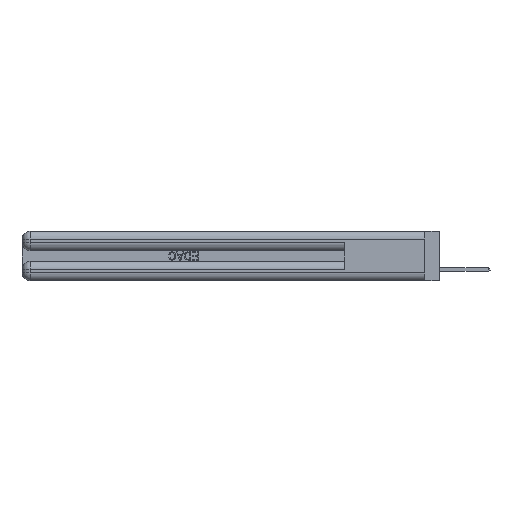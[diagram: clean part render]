
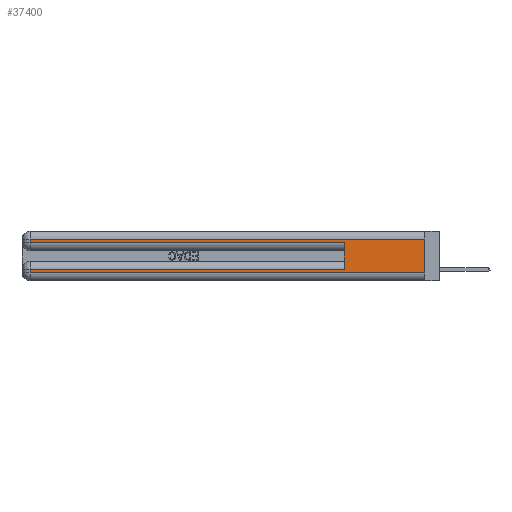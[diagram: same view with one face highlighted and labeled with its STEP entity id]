
A CAD part, left-side view. The second image highlights one B-rep face of the part: STEP entity #37400.
In plain terms, the highlighted planar face has unit normal (-1, 0, 0).
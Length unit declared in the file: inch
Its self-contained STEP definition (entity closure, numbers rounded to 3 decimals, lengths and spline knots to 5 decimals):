
#959 = FACE_OUTER_BOUND ( 'NONE', #41327, .T. ) ;
#1634 = CARTESIAN_POINT ( 'NONE',  ( 0., 2.94, 0.085 ) ) ;
#2557 = DIRECTION ( 'NONE',  ( 0., -1., 0. ) ) ;
#3892 = CARTESIAN_POINT ( 'NONE',  ( 0., 0., 0.285 ) ) ;
#4007 = VERTEX_POINT ( 'NONE', #27231 ) ;
#5048 = CARTESIAN_POINT ( 'NONE',  ( 0., 2.94, 0.06 ) ) ;
#6409 = LINE ( 'NONE', #3892, #15385 ) ;
#7147 = VECTOR ( 'NONE', #18586, 39.37008 ) ;
#7641 = EDGE_CURVE ( 'NONE', #14360, #9346, #18657, .T. ) ;
#8095 = CARTESIAN_POINT ( 'NONE',  ( 0., 0., 0.37 ) ) ;
#8806 = ORIENTED_EDGE ( 'NONE', *, *, #25575, .T. ) ;
#9346 = VERTEX_POINT ( 'NONE', #25909 ) ;
#9997 = ORIENTED_EDGE ( 'NONE', *, *, #52370, .F. ) ;
#11109 = CARTESIAN_POINT ( 'NONE',  ( 0., 0.6, 0.145 ) ) ;
#11208 = LINE ( 'NONE', #42254, #40417 ) ;
#11433 = LINE ( 'NONE', #36937, #41203 ) ;
#12401 = VERTEX_POINT ( 'NONE', #48566 ) ;
#13920 = CARTESIAN_POINT ( 'NONE',  ( 0., 2.94, 0.31 ) ) ;
#14174 = EDGE_CURVE ( 'NONE', #27865, #9346, #31146, .T. ) ;
#14360 = VERTEX_POINT ( 'NONE', #41573 ) ;
#15385 = VECTOR ( 'NONE', #36323, 39.37008 ) ;
#18154 = VERTEX_POINT ( 'NONE', #39111 ) ;
#18579 = VECTOR ( 'NONE', #2557, 39.37008 ) ;
#18586 = DIRECTION ( 'NONE',  ( 0., 0., 1. ) ) ;
#18657 = LINE ( 'NONE', #38219, #36341 ) ;
#19942 = EDGE_CURVE ( 'NONE', #12401, #45869, #11433, .T. ) ;
#20058 = ORIENTED_EDGE ( 'NONE', *, *, #19942, .T. ) ;
#20278 = VECTOR ( 'NONE', #51537, 39.37008 ) ;
#23236 = CARTESIAN_POINT ( 'NONE',  ( 0., 2.94, 0.37 ) ) ;
#23429 = EDGE_CURVE ( 'NONE', #45869, #27865, #37323, .T. ) ;
#23439 = ORIENTED_EDGE ( 'NONE', *, *, #23429, .T. ) ;
#24283 = ORIENTED_EDGE ( 'NONE', *, *, #14174, .T. ) ;
#24435 = DIRECTION ( 'NONE',  ( 0., 0., -1. ) ) ;
#25575 = EDGE_CURVE ( 'NONE', #30558, #4007, #11208, .T. ) ;
#25909 = CARTESIAN_POINT ( 'NONE',  ( 0., 0., 0.06 ) ) ;
#27231 = CARTESIAN_POINT ( 'NONE',  ( 0., 2.94, 0.285 ) ) ;
#27865 = VERTEX_POINT ( 'NONE', #5048 ) ;
#29113 = DIRECTION ( 'NONE',  ( 0., 1., 0. ) ) ;
#29171 = CARTESIAN_POINT ( 'NONE',  ( 0., 0., 0.31 ) ) ;
#29305 = LINE ( 'NONE', #11109, #7147 ) ;
#30222 = ORIENTED_EDGE ( 'NONE', *, *, #47923, .T. ) ;
#30558 = VERTEX_POINT ( 'NONE', #13920 ) ;
#31146 = LINE ( 'NONE', #34938, #18579 ) ;
#32526 = PLANE ( 'NONE',  #49055 ) ;
#34938 = CARTESIAN_POINT ( 'NONE',  ( 0., 0., 0.06 ) ) ;
#36323 = DIRECTION ( 'NONE',  ( 0., -1., 0. ) ) ;
#36341 = VECTOR ( 'NONE', #42694, 39.37008 ) ;
#36937 = CARTESIAN_POINT ( 'NONE',  ( 0., 0., 0.085 ) ) ;
#37323 = LINE ( 'NONE', #23236, #20278 ) ;
#37400 = ADVANCED_FACE ( 'NONE', ( #959 ), #32526, .F. ) ;
#38219 = CARTESIAN_POINT ( 'NONE',  ( 0., 0., 0.37 ) ) ;
#39111 = CARTESIAN_POINT ( 'NONE',  ( 0., 0.6, 0.285 ) ) ;
#40417 = VECTOR ( 'NONE', #50723, 39.37008 ) ;
#41203 = VECTOR ( 'NONE', #29113, 39.37008 ) ;
#41327 = EDGE_LOOP ( 'NONE', ( #42657, #48228, #8806, #30222, #9997, #20058, #23439, #24283 ) ) ;
#41573 = CARTESIAN_POINT ( 'NONE',  ( 0., 0., 0.31 ) ) ;
#42254 = CARTESIAN_POINT ( 'NONE',  ( 0., 2.94, 0.37 ) ) ;
#42657 = ORIENTED_EDGE ( 'NONE', *, *, #7641, .F. ) ;
#42694 = DIRECTION ( 'NONE',  ( 0., 0., -1. ) ) ;
#45191 = DIRECTION ( 'NONE',  ( 0., 1., 0. ) ) ;
#45869 = VERTEX_POINT ( 'NONE', #1634 ) ;
#45940 = VECTOR ( 'NONE', #45191, 39.37008 ) ;
#47244 = LINE ( 'NONE', #29171, #45940 ) ;
#47923 = EDGE_CURVE ( 'NONE', #4007, #18154, #6409, .T. ) ;
#48228 = ORIENTED_EDGE ( 'NONE', *, *, #51582, .T. ) ;
#48566 = CARTESIAN_POINT ( 'NONE',  ( 0., 0.6, 0.085 ) ) ;
#48883 = DIRECTION ( 'NONE',  ( 1., 0., 0. ) ) ;
#49055 = AXIS2_PLACEMENT_3D ( 'NONE', #8095, #48883, #24435 ) ;
#50723 = DIRECTION ( 'NONE',  ( 0., 0., -1. ) ) ;
#51537 = DIRECTION ( 'NONE',  ( 0., 0., -1. ) ) ;
#51582 = EDGE_CURVE ( 'NONE', #14360, #30558, #47244, .T. ) ;
#52370 = EDGE_CURVE ( 'NONE', #12401, #18154, #29305, .T. ) ;
